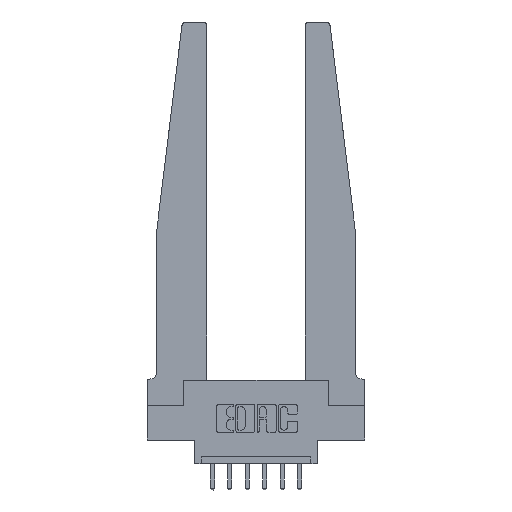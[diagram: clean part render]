
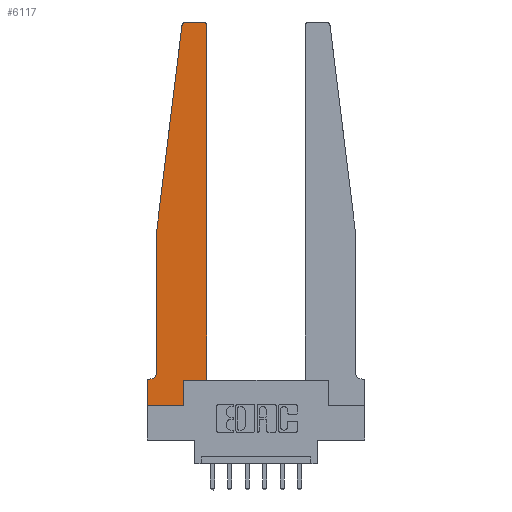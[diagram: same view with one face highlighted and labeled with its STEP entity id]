
A CAD part, top view. The second image highlights one B-rep face of the part: STEP entity #6117.
In plain terms, the highlighted planar face has unit normal (0, 0, 1).
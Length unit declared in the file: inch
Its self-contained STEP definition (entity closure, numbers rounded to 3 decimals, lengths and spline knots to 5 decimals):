
#69 = ORIENTED_EDGE ( 'NONE', *, *, #7607, .T. ) ;
#189 = DIRECTION ( 'NONE',  ( 1., 0., 0. ) ) ;
#383 = CARTESIAN_POINT ( 'NONE',  ( 0.425, 0.18, 0.37 ) ) ;
#472 = AXIS2_PLACEMENT_3D ( 'NONE', #11848, #8718, #189 ) ;
#593 = CARTESIAN_POINT ( 'NONE',  ( 0.24675, 2.72367, 0.37 ) ) ;
#624 = ORIENTED_EDGE ( 'NONE', *, *, #9066, .T. ) ;
#714 = EDGE_CURVE ( 'NONE', #9904, #6010, #13088, .T. ) ;
#927 = CARTESIAN_POINT ( 'NONE',  ( 0.065, 1.25, 0.37 ) ) ;
#938 = CARTESIAN_POINT ( 'NONE',  ( 0.2605, 0., 0.37 ) ) ;
#941 = VERTEX_POINT ( 'NONE', #593 ) ;
#1168 = CARTESIAN_POINT ( 'NONE',  ( 0.2605, 0.18, 0.37 ) ) ;
#1359 = ORIENTED_EDGE ( 'NONE', *, *, #4934, .T. ) ;
#1501 = CARTESIAN_POINT ( 'NONE',  ( 0., 0., 0.37 ) ) ;
#1881 = ORIENTED_EDGE ( 'NONE', *, *, #9955, .T. ) ;
#1995 = LINE ( 'NONE', #4207, #11940 ) ;
#2282 = LINE ( 'NONE', #383, #6965 ) ;
#2452 = VECTOR ( 'NONE', #8317, 39.37008 ) ;
#2608 = DIRECTION ( 'NONE',  ( -1., 0., 0. ) ) ;
#2737 = ORIENTED_EDGE ( 'NONE', *, *, #4713, .T. ) ;
#2949 = CIRCLE ( 'NONE', #10839, 0.05 ) ;
#3147 = CARTESIAN_POINT ( 'NONE',  ( 0., 0.1875, 0.37 ) ) ;
#3179 = VERTEX_POINT ( 'NONE', #3147 ) ;
#3341 = LINE ( 'NONE', #5520, #5382 ) ;
#3458 = EDGE_CURVE ( 'NONE', #3179, #9904, #11142, .T. ) ;
#3557 = DIRECTION ( 'NONE',  ( 1., 0., 0. ) ) ;
#3570 = CARTESIAN_POINT ( 'NONE',  ( 0.2605, 0.18, 0.37 ) ) ;
#3648 = DIRECTION ( 'NONE',  ( 0., 0., 1. ) ) ;
#3877 = VERTEX_POINT ( 'NONE', #13901 ) ;
#4091 = FACE_OUTER_BOUND ( 'NONE', #4142, .T. ) ;
#4142 = EDGE_LOOP ( 'NONE', ( #624, #69, #13207, #2737, #11797, #1359, #11630, #10596, #9072, #13187, #10824, #1881 ) ) ;
#4207 = CARTESIAN_POINT ( 'NONE',  ( 0.065, 1.25, 0.37 ) ) ;
#4340 = DIRECTION ( 'NONE',  ( 0., 1., 0. ) ) ;
#4520 = AXIS2_PLACEMENT_3D ( 'NONE', #12112, #3648, #6823 ) ;
#4540 = VECTOR ( 'NONE', #6035, 39.37008 ) ;
#4713 = EDGE_CURVE ( 'NONE', #11272, #3877, #1995, .T. ) ;
#4812 = CARTESIAN_POINT ( 'NONE',  ( 0.015, 0.2375, 0.37 ) ) ;
#4934 = EDGE_CURVE ( 'NONE', #6300, #3179, #10582, .T. ) ;
#4994 = LINE ( 'NONE', #10177, #11958 ) ;
#5077 = VERTEX_POINT ( 'NONE', #8503 ) ;
#5304 = VERTEX_POINT ( 'NONE', #1168 ) ;
#5382 = VECTOR ( 'NONE', #4340, 39.37008 ) ;
#5520 = CARTESIAN_POINT ( 'NONE',  ( 0.425, 0.18, 0.37 ) ) ;
#5627 = LINE ( 'NONE', #7892, #9430 ) ;
#5804 = DIRECTION ( 'NONE',  ( 0., -1., 0. ) ) ;
#6010 = VERTEX_POINT ( 'NONE', #938 ) ;
#6035 = DIRECTION ( 'NONE',  ( 0., 1., 0. ) ) ;
#6053 = EDGE_CURVE ( 'NONE', #10476, #8409, #3341, .T. ) ;
#6117 = ADVANCED_FACE ( 'NONE', ( #4091 ), #12802, .T. ) ;
#6140 = DIRECTION ( 'NONE',  ( 1., 0., 0. ) ) ;
#6300 = VERTEX_POINT ( 'NONE', #6976 ) ;
#6788 = CIRCLE ( 'NONE', #472, 0.03 ) ;
#6823 = DIRECTION ( 'NONE',  ( 1., 0., 0. ) ) ;
#6965 = VECTOR ( 'NONE', #3557, 39.37008 ) ;
#6976 = CARTESIAN_POINT ( 'NONE',  ( 0.015, 0.1875, 0.37 ) ) ;
#7607 = EDGE_CURVE ( 'NONE', #13402, #941, #6788, .T. ) ;
#7892 = CARTESIAN_POINT ( 'NONE',  ( 0.065, 1.25, 0.37 ) ) ;
#7978 = DIRECTION ( 'NONE',  ( 0., 0., -1. ) ) ;
#8317 = DIRECTION ( 'NONE',  ( -1., 0., 0. ) ) ;
#8409 = VERTEX_POINT ( 'NONE', #9282 ) ;
#8503 = CARTESIAN_POINT ( 'NONE',  ( 0.395, 2.75, 0.37 ) ) ;
#8718 = DIRECTION ( 'NONE',  ( 0., 0., 1. ) ) ;
#8911 = CARTESIAN_POINT ( 'NONE',  ( 0., 0., 0.37 ) ) ;
#9066 = EDGE_CURVE ( 'NONE', #5077, #13402, #4994, .T. ) ;
#9072 = ORIENTED_EDGE ( 'NONE', *, *, #10538, .T. ) ;
#9282 = CARTESIAN_POINT ( 'NONE',  ( 0.425, 2.72, 0.37 ) ) ;
#9424 = DIRECTION ( 'NONE',  ( 0., 0., 1. ) ) ;
#9430 = VECTOR ( 'NONE', #9925, 39.37008 ) ;
#9576 = CARTESIAN_POINT ( 'NONE',  ( 0.065, 0.1875, 0.37 ) ) ;
#9904 = VERTEX_POINT ( 'NONE', #10989 ) ;
#9925 = DIRECTION ( 'NONE',  ( -0.122, -0.992, 0. ) ) ;
#9955 = EDGE_CURVE ( 'NONE', #8409, #5077, #13140, .T. ) ;
#10177 = CARTESIAN_POINT ( 'NONE',  ( 0.25, 2.75, 0.37 ) ) ;
#10296 = VECTOR ( 'NONE', #11106, 39.37008 ) ;
#10372 = EDGE_CURVE ( 'NONE', #3877, #6300, #2949, .T. ) ;
#10391 = DIRECTION ( 'NONE',  ( -1., 0., 0. ) ) ;
#10476 = VERTEX_POINT ( 'NONE', #11991 ) ;
#10538 = EDGE_CURVE ( 'NONE', #6010, #5304, #12331, .T. ) ;
#10582 = LINE ( 'NONE', #9576, #2452 ) ;
#10596 = ORIENTED_EDGE ( 'NONE', *, *, #714, .T. ) ;
#10824 = ORIENTED_EDGE ( 'NONE', *, *, #6053, .T. ) ;
#10839 = AXIS2_PLACEMENT_3D ( 'NONE', #4812, #7978, #2608 ) ;
#10989 = CARTESIAN_POINT ( 'NONE',  ( 0., 0., 0.37 ) ) ;
#11106 = DIRECTION ( 'NONE',  ( 1., 0., 0. ) ) ;
#11142 = LINE ( 'NONE', #1501, #11443 ) ;
#11272 = VERTEX_POINT ( 'NONE', #927 ) ;
#11443 = VECTOR ( 'NONE', #5804, 39.37008 ) ;
#11458 = AXIS2_PLACEMENT_3D ( 'NONE', #11494, #9424, #6140 ) ;
#11494 = CARTESIAN_POINT ( 'NONE',  ( 0., 0.1875, 0.37 ) ) ;
#11578 = EDGE_CURVE ( 'NONE', #941, #11272, #5627, .T. ) ;
#11630 = ORIENTED_EDGE ( 'NONE', *, *, #3458, .T. ) ;
#11797 = ORIENTED_EDGE ( 'NONE', *, *, #10372, .T. ) ;
#11848 = CARTESIAN_POINT ( 'NONE',  ( 0.27653, 2.72, 0.37 ) ) ;
#11940 = VECTOR ( 'NONE', #12865, 39.37008 ) ;
#11958 = VECTOR ( 'NONE', #10391, 39.37008 ) ;
#11991 = CARTESIAN_POINT ( 'NONE',  ( 0.425, 0.18, 0.37 ) ) ;
#12112 = CARTESIAN_POINT ( 'NONE',  ( 0.395, 2.72, 0.37 ) ) ;
#12131 = EDGE_CURVE ( 'NONE', #5304, #10476, #2282, .T. ) ;
#12331 = LINE ( 'NONE', #3570, #4540 ) ;
#12802 = PLANE ( 'NONE',  #11458 ) ;
#12865 = DIRECTION ( 'NONE',  ( 0., -1., 0. ) ) ;
#13088 = LINE ( 'NONE', #8911, #10296 ) ;
#13140 = CIRCLE ( 'NONE', #4520, 0.03 ) ;
#13187 = ORIENTED_EDGE ( 'NONE', *, *, #12131, .T. ) ;
#13207 = ORIENTED_EDGE ( 'NONE', *, *, #11578, .T. ) ;
#13230 = CARTESIAN_POINT ( 'NONE',  ( 0.27653, 2.75, 0.37 ) ) ;
#13402 = VERTEX_POINT ( 'NONE', #13230 ) ;
#13901 = CARTESIAN_POINT ( 'NONE',  ( 0.065, 0.2375, 0.37 ) ) ;
